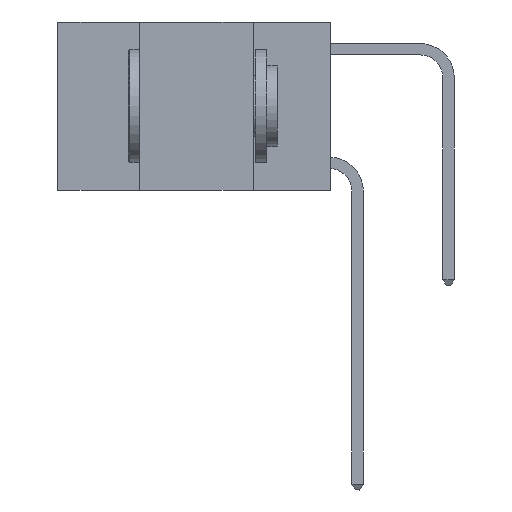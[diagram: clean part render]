
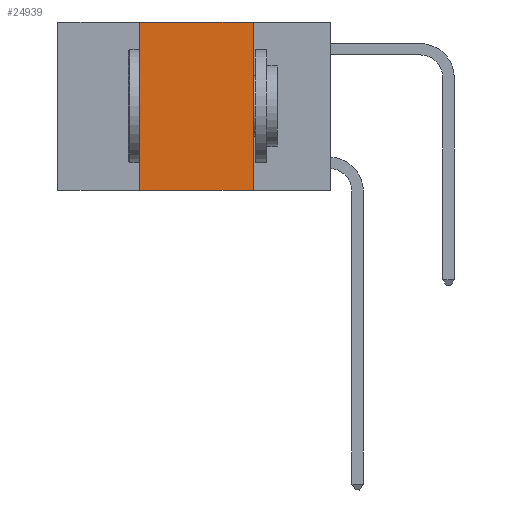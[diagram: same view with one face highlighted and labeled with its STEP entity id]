
A CAD part, left-side view. The second image highlights one B-rep face of the part: STEP entity #24939.
In plain terms, the highlighted planar face has unit normal (-1, 0, 0).
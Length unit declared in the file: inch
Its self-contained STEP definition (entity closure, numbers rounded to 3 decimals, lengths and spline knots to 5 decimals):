
#332 = ORIENTED_EDGE ( 'NONE', *, *, #22925, .F. ) ;
#889 = CARTESIAN_POINT ( 'NONE',  ( 0., 0.17, 0. ) ) ;
#1813 = DIRECTION ( 'NONE',  ( 0., -1., 0. ) ) ;
#2847 = DIRECTION ( 'NONE',  ( 0., 0., -1. ) ) ;
#2902 = PLANE ( 'NONE',  #24627 ) ;
#2909 = VECTOR ( 'NONE', #2847, 39.37008 ) ;
#3780 = CARTESIAN_POINT ( 'NONE',  ( 0., 0.6, 0. ) ) ;
#4348 = ORIENTED_EDGE ( 'NONE', *, *, #24550, .F. ) ;
#4397 = CARTESIAN_POINT ( 'NONE',  ( 0., 0.42, 0. ) ) ;
#5351 = VECTOR ( 'NONE', #1813, 39.37008 ) ;
#5549 = ORIENTED_EDGE ( 'NONE', *, *, #21631, .T. ) ;
#5824 = VERTEX_POINT ( 'NONE', #15607 ) ;
#5952 = CARTESIAN_POINT ( 'NONE',  ( 0., 0.17, 0. ) ) ;
#6344 = DIRECTION ( 'NONE',  ( 0., 0., 1. ) ) ;
#6351 = LINE ( 'NONE', #4397, #11580 ) ;
#6841 = DIRECTION ( 'NONE',  ( 0., 0., -1. ) ) ;
#8131 = LINE ( 'NONE', #889, #2909 ) ;
#9115 = VERTEX_POINT ( 'NONE', #19273 ) ;
#10439 = VECTOR ( 'NONE', #16343, 39.37008 ) ;
#10566 = LINE ( 'NONE', #3780, #5351 ) ;
#11580 = VECTOR ( 'NONE', #6344, 39.37008 ) ;
#12994 = VERTEX_POINT ( 'NONE', #20203 ) ;
#14377 = CARTESIAN_POINT ( 'NONE',  ( 0., 0.6, -0.37 ) ) ;
#15607 = CARTESIAN_POINT ( 'NONE',  ( 0., 0.42, 0. ) ) ;
#16343 = DIRECTION ( 'NONE',  ( 0., -1., 0. ) ) ;
#18196 = FACE_OUTER_BOUND ( 'NONE', #20568, .T. ) ;
#18576 = DIRECTION ( 'NONE',  ( 1., 0., 0. ) ) ;
#19273 = CARTESIAN_POINT ( 'NONE',  ( 0., 0.17, -0.37 ) ) ;
#20203 = CARTESIAN_POINT ( 'NONE',  ( 0., 0.42, -0.37 ) ) ;
#20568 = EDGE_LOOP ( 'NONE', ( #24530, #4348, #332, #5549 ) ) ;
#20863 = LINE ( 'NONE', #14377, #10439 ) ;
#21631 = EDGE_CURVE ( 'NONE', #12994, #9115, #20863, .T. ) ;
#22103 = VERTEX_POINT ( 'NONE', #5952 ) ;
#22925 = EDGE_CURVE ( 'NONE', #12994, #5824, #6351, .T. ) ;
#24233 = EDGE_CURVE ( 'NONE', #22103, #9115, #8131, .T. ) ;
#24395 = CARTESIAN_POINT ( 'NONE',  ( 0., 0.6, 0. ) ) ;
#24530 = ORIENTED_EDGE ( 'NONE', *, *, #24233, .F. ) ;
#24550 = EDGE_CURVE ( 'NONE', #5824, #22103, #10566, .T. ) ;
#24627 = AXIS2_PLACEMENT_3D ( 'NONE', #24395, #18576, #6841 ) ;
#24939 = ADVANCED_FACE ( 'NONE', ( #18196 ), #2902, .F. ) ;
